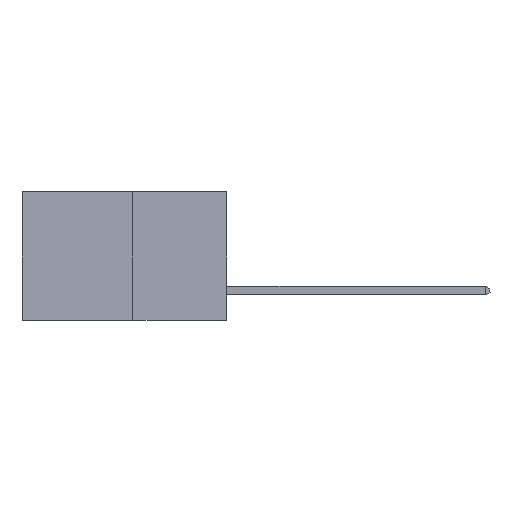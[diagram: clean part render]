
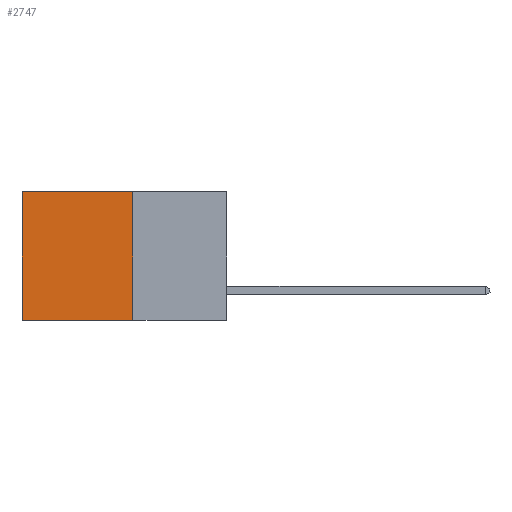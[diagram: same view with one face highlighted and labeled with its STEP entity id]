
A CAD part, left-side view. The second image highlights one B-rep face of the part: STEP entity #2747.
In plain terms, the highlighted planar face has unit normal (-1, 0, 0).
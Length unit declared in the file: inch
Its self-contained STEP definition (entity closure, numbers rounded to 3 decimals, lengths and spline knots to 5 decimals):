
#77 = ORIENTED_EDGE ( 'NONE', *, *, #11421, .T. ) ;
#535 = ORIENTED_EDGE ( 'NONE', *, *, #5683, .F. ) ;
#1125 = FACE_OUTER_BOUND ( 'NONE', #8904, .T. ) ;
#1205 = VECTOR ( 'NONE', #4737, 39.37008 ) ;
#2245 = VERTEX_POINT ( 'NONE', #9198 ) ;
#2747 = ADVANCED_FACE ( 'NONE', ( #1125 ), #5733, .F. ) ;
#2820 = CARTESIAN_POINT ( 'NONE',  ( 0.277, 0.27, -0.37 ) ) ;
#3133 = VERTEX_POINT ( 'NONE', #5961 ) ;
#3143 = VERTEX_POINT ( 'NONE', #5745 ) ;
#3377 = DIRECTION ( 'NONE',  ( 0., 0., -1. ) ) ;
#3734 = DIRECTION ( 'NONE',  ( 0., 0., -1. ) ) ;
#3889 = CARTESIAN_POINT ( 'NONE',  ( 0.277, 0.59, -0.37 ) ) ;
#3960 = LINE ( 'NONE', #8239, #1205 ) ;
#4014 = DIRECTION ( 'NONE',  ( 1., 0., 0. ) ) ;
#4239 = VECTOR ( 'NONE', #3734, 39.37008 ) ;
#4737 = DIRECTION ( 'NONE',  ( 0., 1., 0. ) ) ;
#5001 = CARTESIAN_POINT ( 'NONE',  ( 0.277, 0.27, -0.37 ) ) ;
#5413 = ORIENTED_EDGE ( 'NONE', *, *, #10996, .T. ) ;
#5683 = EDGE_CURVE ( 'NONE', #2245, #9964, #6328, .T. ) ;
#5733 = PLANE ( 'NONE',  #10457 ) ;
#5745 = CARTESIAN_POINT ( 'NONE',  ( 0.277, 0.59, 0. ) ) ;
#5749 = LINE ( 'NONE', #7744, #7842 ) ;
#5961 = CARTESIAN_POINT ( 'NONE',  ( 0.277, 0.59, -0.37 ) ) ;
#6328 = LINE ( 'NONE', #2820, #4239 ) ;
#6375 = EDGE_CURVE ( 'NONE', #9964, #3133, #3960, .T. ) ;
#6386 = ORIENTED_EDGE ( 'NONE', *, *, #6375, .F. ) ;
#7577 = CARTESIAN_POINT ( 'NONE',  ( 0.277, 0.27, -0.37 ) ) ;
#7744 = CARTESIAN_POINT ( 'NONE',  ( 0.277, 0.27, 0. ) ) ;
#7842 = VECTOR ( 'NONE', #10314, 39.37008 ) ;
#8239 = CARTESIAN_POINT ( 'NONE',  ( 0.277, 0.27, -0.37 ) ) ;
#8641 = LINE ( 'NONE', #3889, #10617 ) ;
#8904 = EDGE_LOOP ( 'NONE', ( #77, #6386, #535, #5413 ) ) ;
#9156 = DIRECTION ( 'NONE',  ( 0., 0., -1. ) ) ;
#9198 = CARTESIAN_POINT ( 'NONE',  ( 0.277, 0.27, 0. ) ) ;
#9964 = VERTEX_POINT ( 'NONE', #7577 ) ;
#10314 = DIRECTION ( 'NONE',  ( 0., 1., 0. ) ) ;
#10457 = AXIS2_PLACEMENT_3D ( 'NONE', #5001, #4014, #3377 ) ;
#10617 = VECTOR ( 'NONE', #9156, 39.37008 ) ;
#10996 = EDGE_CURVE ( 'NONE', #2245, #3143, #5749, .T. ) ;
#11421 = EDGE_CURVE ( 'NONE', #3143, #3133, #8641, .T. ) ;
